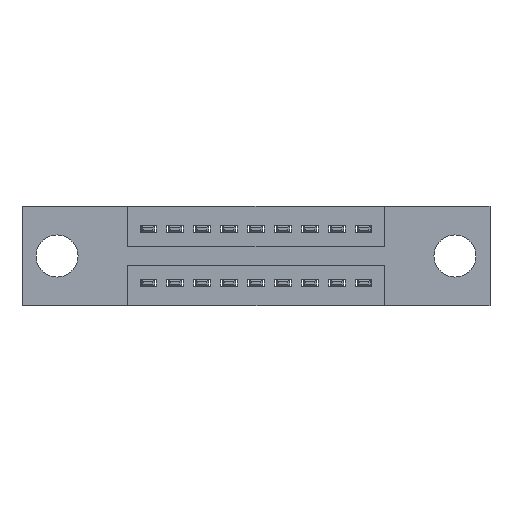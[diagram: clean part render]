
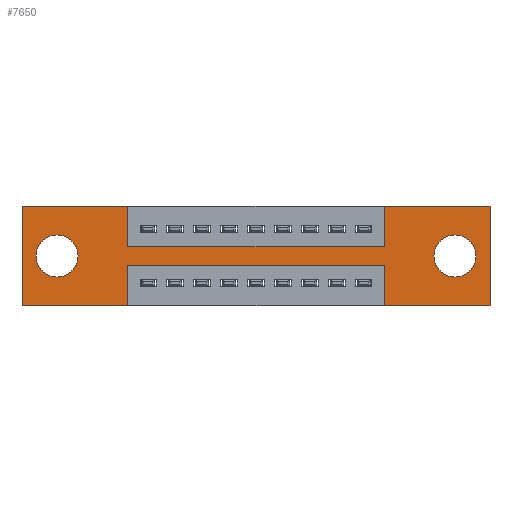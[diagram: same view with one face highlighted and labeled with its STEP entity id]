
A CAD part, front view. The second image highlights one B-rep face of the part: STEP entity #7650.
In plain terms, the highlighted planar face has unit normal (0, -1, 0).
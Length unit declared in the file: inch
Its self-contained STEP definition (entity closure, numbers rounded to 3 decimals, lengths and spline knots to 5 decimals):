
#30 = CARTESIAN_POINT ( 'NONE',  ( 0., 0., -0.37 ) ) ;
#68 = EDGE_CURVE ( 'NONE', #10618, #342, #7868, .T. ) ;
#167 = VECTOR ( 'NONE', #10214, 39.37008 ) ;
#192 = EDGE_CURVE ( 'NONE', #2120, #1803, #10229, .T. ) ;
#201 = CARTESIAN_POINT ( 'NONE',  ( 1.735, 0., 0. ) ) ;
#262 = EDGE_CURVE ( 'NONE', #2567, #7744, #2835, .T. ) ;
#342 = VERTEX_POINT ( 'NONE', #5911 ) ;
#442 = ORIENTED_EDGE ( 'NONE', *, *, #660, .F. ) ;
#573 = VERTEX_POINT ( 'NONE', #4680 ) ;
#578 = VECTOR ( 'NONE', #9461, 39.37008 ) ;
#646 = CARTESIAN_POINT ( 'NONE',  ( 1.3425, 0., 0. ) ) ;
#660 = EDGE_CURVE ( 'NONE', #342, #2567, #3482, .T. ) ;
#689 = AXIS2_PLACEMENT_3D ( 'NONE', #30, #3616, #5352 ) ;
#730 = DIRECTION ( 'NONE',  ( 0., 0., 1. ) ) ;
#874 = CARTESIAN_POINT ( 'NONE',  ( 1.605, 0., -0.185 ) ) ;
#1055 = EDGE_LOOP ( 'NONE', ( #7582, #9313, #1587, #1129, #6452, #10178, #1483, #4691, #6404, #442, #8713, #4790 ) ) ;
#1105 = CARTESIAN_POINT ( 'NONE',  ( 0.3925, 0., 0. ) ) ;
#1129 = ORIENTED_EDGE ( 'NONE', *, *, #3756, .F. ) ;
#1292 = LINE ( 'NONE', #11050, #10334 ) ;
#1472 = CARTESIAN_POINT ( 'NONE',  ( 0.13, 0., -0.185 ) ) ;
#1483 = ORIENTED_EDGE ( 'NONE', *, *, #10776, .F. ) ;
#1538 = DIRECTION ( 'NONE',  ( 0., 0., -1. ) ) ;
#1587 = ORIENTED_EDGE ( 'NONE', *, *, #3698, .F. ) ;
#1635 = CARTESIAN_POINT ( 'NONE',  ( 0.13, 0., -0.107 ) ) ;
#1649 = LINE ( 'NONE', #7415, #7522 ) ;
#1799 = CARTESIAN_POINT ( 'NONE',  ( 1.735, 0., -0.37 ) ) ;
#1803 = VERTEX_POINT ( 'NONE', #11032 ) ;
#1820 = VECTOR ( 'NONE', #2752, 39.37008 ) ;
#1885 = CARTESIAN_POINT ( 'NONE',  ( 0., 0., -0.37 ) ) ;
#2120 = VERTEX_POINT ( 'NONE', #8045 ) ;
#2137 = FACE_BOUND ( 'NONE', #8736, .T. ) ;
#2225 = ORIENTED_EDGE ( 'NONE', *, *, #6665, .T. ) ;
#2284 = CIRCLE ( 'NONE', #10583, 0.078 ) ;
#2341 = CIRCLE ( 'NONE', #9677, 0.078 ) ;
#2490 = VERTEX_POINT ( 'NONE', #3708 ) ;
#2567 = VERTEX_POINT ( 'NONE', #1105 ) ;
#2752 = DIRECTION ( 'NONE',  ( -1., 0., 0. ) ) ;
#2835 = LINE ( 'NONE', #6735, #9815 ) ;
#2840 = EDGE_CURVE ( 'NONE', #10978, #9131, #10167, .T. ) ;
#2881 = EDGE_LOOP ( 'NONE', ( #9607, #2225 ) ) ;
#2979 = CARTESIAN_POINT ( 'NONE',  ( 0., 0., 0. ) ) ;
#3052 = EDGE_CURVE ( 'NONE', #7068, #10618, #7665, .T. ) ;
#3482 = LINE ( 'NONE', #8247, #4821 ) ;
#3568 = DIRECTION ( 'NONE',  ( 0., 1., 0. ) ) ;
#3616 = DIRECTION ( 'NONE',  ( 0., -1., 0. ) ) ;
#3698 = EDGE_CURVE ( 'NONE', #2490, #573, #4219, .T. ) ;
#3708 = CARTESIAN_POINT ( 'NONE',  ( 1.3425, 0., -0.37 ) ) ;
#3739 = CIRCLE ( 'NONE', #9798, 0.078 ) ;
#3756 = EDGE_CURVE ( 'NONE', #9131, #2490, #1649, .T. ) ;
#3801 = CARTESIAN_POINT ( 'NONE',  ( 0., 0., 0. ) ) ;
#3827 = PLANE ( 'NONE',  #689 ) ;
#3977 = CARTESIAN_POINT ( 'NONE',  ( 1.3425, 0., -0.37 ) ) ;
#4026 = FACE_OUTER_BOUND ( 'NONE', #1055, .T. ) ;
#4087 = AXIS2_PLACEMENT_3D ( 'NONE', #874, #3568, #9693 ) ;
#4219 = LINE ( 'NONE', #3977, #6116 ) ;
#4444 = DIRECTION ( 'NONE',  ( 0., 0., -1. ) ) ;
#4562 = VECTOR ( 'NONE', #9104, 39.37008 ) ;
#4674 = CARTESIAN_POINT ( 'NONE',  ( 0.3925, 0., -0.15 ) ) ;
#4680 = CARTESIAN_POINT ( 'NONE',  ( 1.3425, 0., -0.22 ) ) ;
#4691 = ORIENTED_EDGE ( 'NONE', *, *, #8594, .F. ) ;
#4790 = ORIENTED_EDGE ( 'NONE', *, *, #3052, .F. ) ;
#4820 = DIRECTION ( 'NONE',  ( -1., 0., 0. ) ) ;
#4821 = VECTOR ( 'NONE', #10963, 39.37008 ) ;
#5120 = CARTESIAN_POINT ( 'NONE',  ( 0.3925, 0., -0.15 ) ) ;
#5204 = VERTEX_POINT ( 'NONE', #10123 ) ;
#5352 = DIRECTION ( 'NONE',  ( 0., 0., -1. ) ) ;
#5435 = CARTESIAN_POINT ( 'NONE',  ( 1.3425, 0., -0.15 ) ) ;
#5460 = CARTESIAN_POINT ( 'NONE',  ( 1.605, 0., -0.185 ) ) ;
#5629 = CARTESIAN_POINT ( 'NONE',  ( 0.3925, 0., -0.37 ) ) ;
#5789 = DIRECTION ( 'NONE',  ( 0., 0., 1. ) ) ;
#5911 = CARTESIAN_POINT ( 'NONE',  ( 0., 0., 0. ) ) ;
#6116 = VECTOR ( 'NONE', #5789, 39.37008 ) ;
#6126 = LINE ( 'NONE', #5629, #10704 ) ;
#6143 = DIRECTION ( 'NONE',  ( 0., 0., 1. ) ) ;
#6395 = CARTESIAN_POINT ( 'NONE',  ( 0., 0., -0.37 ) ) ;
#6404 = ORIENTED_EDGE ( 'NONE', *, *, #262, .F. ) ;
#6452 = ORIENTED_EDGE ( 'NONE', *, *, #2840, .F. ) ;
#6523 = CARTESIAN_POINT ( 'NONE',  ( 0.3925, 0., -0.37 ) ) ;
#6664 = DIRECTION ( 'NONE',  ( -1., 0., 0. ) ) ;
#6665 = EDGE_CURVE ( 'NONE', #5204, #8159, #2284, .T. ) ;
#6735 = CARTESIAN_POINT ( 'NONE',  ( 0.3925, 0., 0. ) ) ;
#6965 = DIRECTION ( 'NONE',  ( 1., 0., 0. ) ) ;
#7042 = VECTOR ( 'NONE', #6965, 39.37008 ) ;
#7068 = VERTEX_POINT ( 'NONE', #6523 ) ;
#7209 = FACE_BOUND ( 'NONE', #2881, .T. ) ;
#7415 = CARTESIAN_POINT ( 'NONE',  ( 0., 0., -0.37 ) ) ;
#7509 = EDGE_CURVE ( 'NONE', #10440, #10978, #9813, .T. ) ;
#7522 = VECTOR ( 'NONE', #4820, 39.37008 ) ;
#7582 = ORIENTED_EDGE ( 'NONE', *, *, #11191, .F. ) ;
#7650 = ADVANCED_FACE ( 'NONE', ( #2137, #7209, #4026 ), #3827, .T. ) ;
#7665 = LINE ( 'NONE', #1885, #1820 ) ;
#7666 = ORIENTED_EDGE ( 'NONE', *, *, #8683, .T. ) ;
#7744 = VERTEX_POINT ( 'NONE', #4674 ) ;
#7868 = LINE ( 'NONE', #3801, #9265 ) ;
#8045 = CARTESIAN_POINT ( 'NONE',  ( 1.605, 0., -0.263 ) ) ;
#8159 = VERTEX_POINT ( 'NONE', #1635 ) ;
#8247 = CARTESIAN_POINT ( 'NONE',  ( 0., 0., 0. ) ) ;
#8338 = EDGE_CURVE ( 'NONE', #573, #8850, #1292, .T. ) ;
#8366 = DIRECTION ( 'NONE',  ( 0., 1., 0. ) ) ;
#8594 = EDGE_CURVE ( 'NONE', #7744, #10882, #10195, .T. ) ;
#8683 = EDGE_CURVE ( 'NONE', #1803, #2120, #3739, .T. ) ;
#8713 = ORIENTED_EDGE ( 'NONE', *, *, #68, .F. ) ;
#8736 = EDGE_LOOP ( 'NONE', ( #7666, #10266 ) ) ;
#8850 = VERTEX_POINT ( 'NONE', #10805 ) ;
#8885 = DIRECTION ( 'NONE',  ( 0., 1., 0. ) ) ;
#9098 = DIRECTION ( 'NONE',  ( 0., 0., -1. ) ) ;
#9104 = DIRECTION ( 'NONE',  ( 1., 0., 0. ) ) ;
#9131 = VERTEX_POINT ( 'NONE', #1799 ) ;
#9265 = VECTOR ( 'NONE', #730, 39.37008 ) ;
#9313 = ORIENTED_EDGE ( 'NONE', *, *, #8338, .F. ) ;
#9445 = LINE ( 'NONE', #646, #167 ) ;
#9461 = DIRECTION ( 'NONE',  ( 0., 0., -1. ) ) ;
#9607 = ORIENTED_EDGE ( 'NONE', *, *, #11202, .T. ) ;
#9665 = DIRECTION ( 'NONE',  ( 0., 1., 0. ) ) ;
#9677 = AXIS2_PLACEMENT_3D ( 'NONE', #10125, #8366, #11082 ) ;
#9693 = DIRECTION ( 'NONE',  ( 0., 0., -1. ) ) ;
#9798 = AXIS2_PLACEMENT_3D ( 'NONE', #5460, #8885, #4444 ) ;
#9813 = LINE ( 'NONE', #2979, #4562 ) ;
#9815 = VECTOR ( 'NONE', #1538, 39.37008 ) ;
#10123 = CARTESIAN_POINT ( 'NONE',  ( 0.13, 0., -0.263 ) ) ;
#10125 = CARTESIAN_POINT ( 'NONE',  ( 0.13, 0., -0.185 ) ) ;
#10167 = LINE ( 'NONE', #11012, #578 ) ;
#10178 = ORIENTED_EDGE ( 'NONE', *, *, #7509, .F. ) ;
#10195 = LINE ( 'NONE', #5120, #7042 ) ;
#10214 = DIRECTION ( 'NONE',  ( 0., 0., 1. ) ) ;
#10229 = CIRCLE ( 'NONE', #4087, 0.078 ) ;
#10266 = ORIENTED_EDGE ( 'NONE', *, *, #192, .T. ) ;
#10334 = VECTOR ( 'NONE', #6664, 39.37008 ) ;
#10440 = VERTEX_POINT ( 'NONE', #10900 ) ;
#10583 = AXIS2_PLACEMENT_3D ( 'NONE', #1472, #9665, #6143 ) ;
#10618 = VERTEX_POINT ( 'NONE', #6395 ) ;
#10704 = VECTOR ( 'NONE', #9098, 39.37008 ) ;
#10776 = EDGE_CURVE ( 'NONE', #10882, #10440, #9445, .T. ) ;
#10805 = CARTESIAN_POINT ( 'NONE',  ( 0.3925, 0., -0.22 ) ) ;
#10882 = VERTEX_POINT ( 'NONE', #5435 ) ;
#10900 = CARTESIAN_POINT ( 'NONE',  ( 1.3425, 0., 0. ) ) ;
#10963 = DIRECTION ( 'NONE',  ( 1., 0., 0. ) ) ;
#10978 = VERTEX_POINT ( 'NONE', #201 ) ;
#11012 = CARTESIAN_POINT ( 'NONE',  ( 1.735, 0., 0. ) ) ;
#11032 = CARTESIAN_POINT ( 'NONE',  ( 1.605, 0., -0.107 ) ) ;
#11050 = CARTESIAN_POINT ( 'NONE',  ( 0.3925, 0., -0.22 ) ) ;
#11082 = DIRECTION ( 'NONE',  ( 0., 0., 1. ) ) ;
#11191 = EDGE_CURVE ( 'NONE', #8850, #7068, #6126, .T. ) ;
#11202 = EDGE_CURVE ( 'NONE', #8159, #5204, #2341, .T. ) ;
